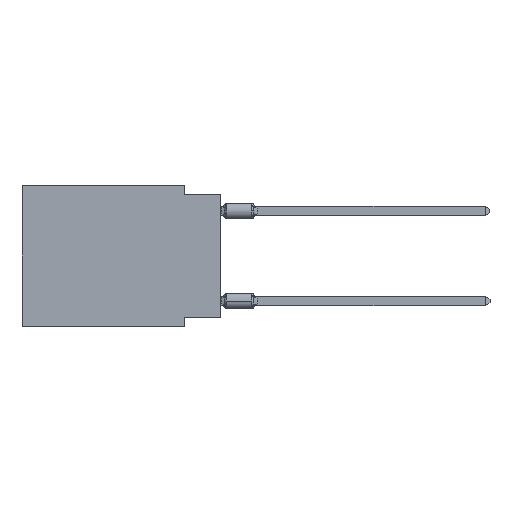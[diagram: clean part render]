
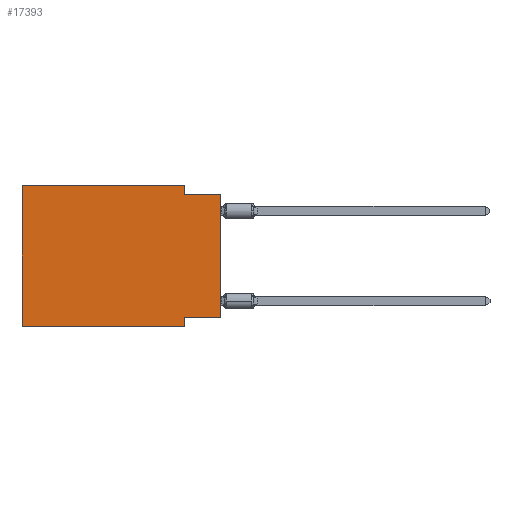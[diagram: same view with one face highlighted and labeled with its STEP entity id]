
A CAD part, left-side view. The second image highlights one B-rep face of the part: STEP entity #17393.
In plain terms, the highlighted planar face has unit normal (-1, 0, 0).
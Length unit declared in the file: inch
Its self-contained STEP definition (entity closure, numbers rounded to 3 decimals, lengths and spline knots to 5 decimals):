
#343 = LINE ( 'NONE', #20553, #3160 ) ;
#1086 = VERTEX_POINT ( 'NONE', #10103 ) ;
#1892 = CARTESIAN_POINT ( 'NONE',  ( 0., 0.55, -0.39 ) ) ;
#2080 = ORIENTED_EDGE ( 'NONE', *, *, #6110, .F. ) ;
#2185 = DIRECTION ( 'NONE',  ( 0., 0., -1. ) ) ;
#2190 = CARTESIAN_POINT ( 'NONE',  ( 0., 0.1, -0.025 ) ) ;
#2297 = LINE ( 'NONE', #6098, #20482 ) ;
#2865 = ORIENTED_EDGE ( 'NONE', *, *, #5187, .T. ) ;
#3062 = VECTOR ( 'NONE', #9746, 39.37008 ) ;
#3148 = EDGE_CURVE ( 'NONE', #18155, #11046, #7021, .T. ) ;
#3160 = VECTOR ( 'NONE', #18716, 39.37008 ) ;
#3238 = VECTOR ( 'NONE', #8860, 39.37008 ) ;
#3239 = CARTESIAN_POINT ( 'NONE',  ( 0., 0.55, 0. ) ) ;
#3489 = FACE_OUTER_BOUND ( 'NONE', #17400, .T. ) ;
#3757 = DIRECTION ( 'NONE',  ( 0., -1., 0. ) ) ;
#4416 = LINE ( 'NONE', #19121, #10812 ) ;
#5187 = EDGE_CURVE ( 'NONE', #17470, #1086, #16755, .T. ) ;
#6098 = CARTESIAN_POINT ( 'NONE',  ( 0., 0.1, 0. ) ) ;
#6110 = EDGE_CURVE ( 'NONE', #18990, #11046, #4416, .T. ) ;
#6702 = LINE ( 'NONE', #18069, #7012 ) ;
#7012 = VECTOR ( 'NONE', #3757, 39.37008 ) ;
#7021 = LINE ( 'NONE', #1892, #3238 ) ;
#7135 = CARTESIAN_POINT ( 'NONE',  ( 0., 0.1, -0.365 ) ) ;
#7527 = VECTOR ( 'NONE', #23968, 39.37008 ) ;
#8860 = DIRECTION ( 'NONE',  ( 0., -1., 0. ) ) ;
#9746 = DIRECTION ( 'NONE',  ( 0., -1., 0. ) ) ;
#10103 = CARTESIAN_POINT ( 'NONE',  ( 0., 0., -0.025 ) ) ;
#10812 = VECTOR ( 'NONE', #19238, 39.37008 ) ;
#10973 = CARTESIAN_POINT ( 'NONE',  ( 0., 0.55, 0. ) ) ;
#11046 = VERTEX_POINT ( 'NONE', #20766 ) ;
#11111 = AXIS2_PLACEMENT_3D ( 'NONE', #10973, #16707, #11223 ) ;
#11223 = DIRECTION ( 'NONE',  ( 0., 0., -1. ) ) ;
#12100 = CARTESIAN_POINT ( 'NONE',  ( 0., 0.55, 0. ) ) ;
#12124 = EDGE_CURVE ( 'NONE', #12237, #19931, #15632, .T. ) ;
#12237 = VERTEX_POINT ( 'NONE', #3239 ) ;
#12705 = ORIENTED_EDGE ( 'NONE', *, *, #20103, .F. ) ;
#13054 = CARTESIAN_POINT ( 'NONE',  ( 0., 0., -0.365 ) ) ;
#13475 = EDGE_CURVE ( 'NONE', #18155, #12237, #16007, .T. ) ;
#13570 = EDGE_CURVE ( 'NONE', #24183, #1086, #6702, .T. ) ;
#13583 = ORIENTED_EDGE ( 'NONE', *, *, #13570, .F. ) ;
#14429 = CARTESIAN_POINT ( 'NONE',  ( 0., 0.1, 0. ) ) ;
#14512 = PLANE ( 'NONE',  #11111 ) ;
#14896 = ORIENTED_EDGE ( 'NONE', *, *, #3148, .T. ) ;
#15463 = ORIENTED_EDGE ( 'NONE', *, *, #13475, .F. ) ;
#15632 = LINE ( 'NONE', #17696, #3062 ) ;
#16007 = LINE ( 'NONE', #12100, #18359 ) ;
#16246 = DIRECTION ( 'NONE',  ( 0., 0., 1. ) ) ;
#16283 = CARTESIAN_POINT ( 'NONE',  ( 0., 0., 0. ) ) ;
#16707 = DIRECTION ( 'NONE',  ( 1., 0., 0. ) ) ;
#16755 = LINE ( 'NONE', #16283, #7527 ) ;
#17393 = ADVANCED_FACE ( 'NONE', ( #3489 ), #14512, .F. ) ;
#17400 = EDGE_LOOP ( 'NONE', ( #2865, #13583, #19090, #20697, #15463, #14896, #2080, #12705 ) ) ;
#17470 = VERTEX_POINT ( 'NONE', #13054 ) ;
#17696 = CARTESIAN_POINT ( 'NONE',  ( 0., 0.55, 0. ) ) ;
#18069 = CARTESIAN_POINT ( 'NONE',  ( 0., 0., -0.025 ) ) ;
#18155 = VERTEX_POINT ( 'NONE', #23283 ) ;
#18359 = VECTOR ( 'NONE', #16246, 39.37008 ) ;
#18716 = DIRECTION ( 'NONE',  ( 0., 1., 0. ) ) ;
#18990 = VERTEX_POINT ( 'NONE', #7135 ) ;
#19090 = ORIENTED_EDGE ( 'NONE', *, *, #21213, .F. ) ;
#19121 = CARTESIAN_POINT ( 'NONE',  ( 0., 0.1, -0.39 ) ) ;
#19238 = DIRECTION ( 'NONE',  ( 0., 0., -1. ) ) ;
#19931 = VERTEX_POINT ( 'NONE', #14429 ) ;
#20103 = EDGE_CURVE ( 'NONE', #17470, #18990, #343, .T. ) ;
#20482 = VECTOR ( 'NONE', #2185, 39.37008 ) ;
#20553 = CARTESIAN_POINT ( 'NONE',  ( 0., 0., -0.365 ) ) ;
#20697 = ORIENTED_EDGE ( 'NONE', *, *, #12124, .F. ) ;
#20766 = CARTESIAN_POINT ( 'NONE',  ( 0., 0.1, -0.39 ) ) ;
#21213 = EDGE_CURVE ( 'NONE', #19931, #24183, #2297, .T. ) ;
#23283 = CARTESIAN_POINT ( 'NONE',  ( 0., 0.55, -0.39 ) ) ;
#23968 = DIRECTION ( 'NONE',  ( 0., 0., 1. ) ) ;
#24183 = VERTEX_POINT ( 'NONE', #2190 ) ;
